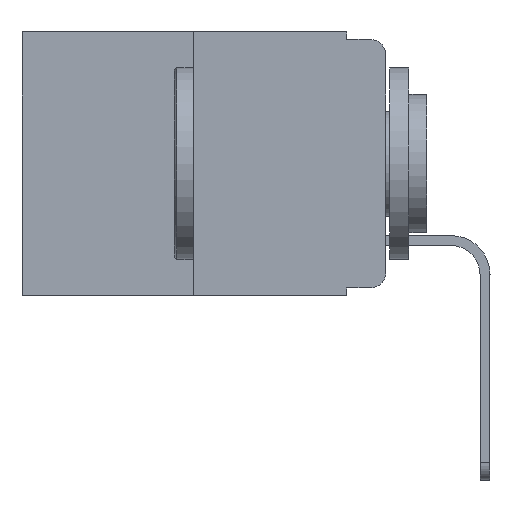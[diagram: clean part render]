
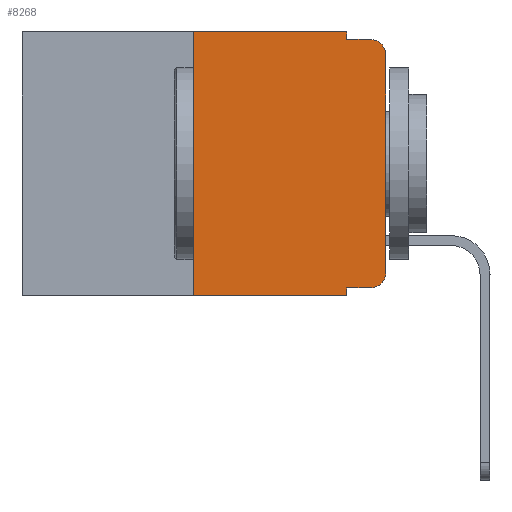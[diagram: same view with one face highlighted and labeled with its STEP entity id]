
A CAD part, left-side view. The second image highlights one B-rep face of the part: STEP entity #8268.
In plain terms, the highlighted planar face has unit normal (-1, 0, 0).
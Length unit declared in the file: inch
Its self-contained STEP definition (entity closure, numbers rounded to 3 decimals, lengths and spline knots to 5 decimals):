
#464 = VERTEX_POINT ( 'NONE', #1537 ) ;
#758 = LINE ( 'NONE', #13825, #1672 ) ;
#880 = CARTESIAN_POINT ( 'NONE',  ( 0., 0.473, 0. ) ) ;
#908 = VERTEX_POINT ( 'NONE', #15043 ) ;
#945 = CARTESIAN_POINT ( 'NONE',  ( 0., 0.02, -0.333 ) ) ;
#1192 = EDGE_CURVE ( 'NONE', #5458, #13924, #758, .T. ) ;
#1350 = DIRECTION ( 'NONE',  ( 0., 0., -1. ) ) ;
#1537 = CARTESIAN_POINT ( 'NONE',  ( 0., 0.25, 0. ) ) ;
#1672 = VECTOR ( 'NONE', #14002, 39.37008 ) ;
#1938 = AXIS2_PLACEMENT_3D ( 'NONE', #14239, #8395, #9851 ) ;
#2137 = VECTOR ( 'NONE', #3473, 39.37008 ) ;
#2298 = EDGE_CURVE ( 'NONE', #14785, #3021, #7307, .T. ) ;
#2560 = EDGE_LOOP ( 'NONE', ( #3801, #17236, #14480, #9229, #12953, #16369, #15485, #13216, #4757, #17441 ) ) ;
#2605 = DIRECTION ( 'NONE',  ( 0., 0., 1. ) ) ;
#2794 = CARTESIAN_POINT ( 'NONE',  ( 0., 0.25, 0. ) ) ;
#3021 = VERTEX_POINT ( 'NONE', #3515 ) ;
#3204 = EDGE_CURVE ( 'NONE', #17879, #13924, #7971, .T. ) ;
#3473 = DIRECTION ( 'NONE',  ( 0., -1., 0. ) ) ;
#3506 = DIRECTION ( 'NONE',  ( 0., 0., 1. ) ) ;
#3515 = CARTESIAN_POINT ( 'NONE',  ( 0., 0.051, -0.01 ) ) ;
#3706 = CARTESIAN_POINT ( 'NONE',  ( 0., 0.051, 0. ) ) ;
#3801 = ORIENTED_EDGE ( 'NONE', *, *, #15115, .T. ) ;
#4421 = CARTESIAN_POINT ( 'NONE',  ( 0., 0.473, 0. ) ) ;
#4757 = ORIENTED_EDGE ( 'NONE', *, *, #10161, .T. ) ;
#4852 = CARTESIAN_POINT ( 'NONE',  ( 0., 0., 0. ) ) ;
#5458 = VERTEX_POINT ( 'NONE', #14608 ) ;
#5532 = LINE ( 'NONE', #880, #13681 ) ;
#5743 = CARTESIAN_POINT ( 'NONE',  ( 0., 0.051, -0.343 ) ) ;
#5960 = EDGE_CURVE ( 'NONE', #908, #10030, #6945, .T. ) ;
#6453 = EDGE_CURVE ( 'NONE', #15244, #16633, #11259, .T. ) ;
#6795 = CARTESIAN_POINT ( 'NONE',  ( 0., 0.473, -0.343 ) ) ;
#6925 = DIRECTION ( 'NONE',  ( 0., -1., 0. ) ) ;
#6945 = CIRCLE ( 'NONE', #8430, 0.02 ) ;
#7133 = DIRECTION ( 'NONE',  ( -1., 0., 0. ) ) ;
#7249 = CARTESIAN_POINT ( 'NONE',  ( 0., 0.051, 0. ) ) ;
#7307 = LINE ( 'NONE', #3706, #8691 ) ;
#7355 = EDGE_CURVE ( 'NONE', #3021, #10030, #13060, .T. ) ;
#7376 = DIRECTION ( 'NONE',  ( 1., 0., 0. ) ) ;
#7581 = FACE_OUTER_BOUND ( 'NONE', #2560, .T. ) ;
#7971 = LINE ( 'NONE', #6795, #17954 ) ;
#8268 = ADVANCED_FACE ( 'NONE', ( #7581 ), #13099, .F. ) ;
#8395 = DIRECTION ( 'NONE',  ( -1., 0., 0. ) ) ;
#8430 = AXIS2_PLACEMENT_3D ( 'NONE', #8550, #7133, #1350 ) ;
#8550 = CARTESIAN_POINT ( 'NONE',  ( 0., 0.02, -0.03 ) ) ;
#8691 = VECTOR ( 'NONE', #10665, 39.37008 ) ;
#9124 = VECTOR ( 'NONE', #15136, 39.37008 ) ;
#9229 = ORIENTED_EDGE ( 'NONE', *, *, #2298, .F. ) ;
#9851 = DIRECTION ( 'NONE',  ( 0., 0., -1. ) ) ;
#10030 = VERTEX_POINT ( 'NONE', #16296 ) ;
#10161 = EDGE_CURVE ( 'NONE', #5458, #15244, #13651, .T. ) ;
#10665 = DIRECTION ( 'NONE',  ( 0., 0., -1. ) ) ;
#11041 = DIRECTION ( 'NONE',  ( 0., -1., 0. ) ) ;
#11259 = CIRCLE ( 'NONE', #1938, 0.02 ) ;
#11471 = VECTOR ( 'NONE', #2605, 39.37008 ) ;
#12383 = CARTESIAN_POINT ( 'NONE',  ( 0., 0.051, -0.333 ) ) ;
#12953 = ORIENTED_EDGE ( 'NONE', *, *, #15248, .F. ) ;
#13060 = LINE ( 'NONE', #13817, #2137 ) ;
#13099 = PLANE ( 'NONE',  #16725 ) ;
#13175 = EDGE_CURVE ( 'NONE', #17879, #464, #17177, .T. ) ;
#13216 = ORIENTED_EDGE ( 'NONE', *, *, #1192, .F. ) ;
#13651 = LINE ( 'NONE', #12383, #9124 ) ;
#13681 = VECTOR ( 'NONE', #11041, 39.37008 ) ;
#13817 = CARTESIAN_POINT ( 'NONE',  ( 0., 0.051, -0.01 ) ) ;
#13825 = CARTESIAN_POINT ( 'NONE',  ( 0., 0.051, 0. ) ) ;
#13924 = VERTEX_POINT ( 'NONE', #5743 ) ;
#14002 = DIRECTION ( 'NONE',  ( 0., 0., -1. ) ) ;
#14239 = CARTESIAN_POINT ( 'NONE',  ( 0., 0.02, -0.313 ) ) ;
#14480 = ORIENTED_EDGE ( 'NONE', *, *, #7355, .F. ) ;
#14572 = DIRECTION ( 'NONE',  ( 0., 0., -1. ) ) ;
#14608 = CARTESIAN_POINT ( 'NONE',  ( 0., 0.051, -0.333 ) ) ;
#14785 = VERTEX_POINT ( 'NONE', #7249 ) ;
#14844 = VECTOR ( 'NONE', #3506, 39.37008 ) ;
#15043 = CARTESIAN_POINT ( 'NONE',  ( 0., 0., -0.03 ) ) ;
#15115 = EDGE_CURVE ( 'NONE', #16633, #908, #17787, .T. ) ;
#15136 = DIRECTION ( 'NONE',  ( 0., -1., 0. ) ) ;
#15244 = VERTEX_POINT ( 'NONE', #945 ) ;
#15248 = EDGE_CURVE ( 'NONE', #464, #14785, #5532, .T. ) ;
#15485 = ORIENTED_EDGE ( 'NONE', *, *, #3204, .T. ) ;
#16296 = CARTESIAN_POINT ( 'NONE',  ( 0., 0.02, -0.01 ) ) ;
#16369 = ORIENTED_EDGE ( 'NONE', *, *, #13175, .F. ) ;
#16633 = VERTEX_POINT ( 'NONE', #18744 ) ;
#16725 = AXIS2_PLACEMENT_3D ( 'NONE', #4421, #7376, #14572 ) ;
#17177 = LINE ( 'NONE', #2794, #11471 ) ;
#17236 = ORIENTED_EDGE ( 'NONE', *, *, #5960, .T. ) ;
#17441 = ORIENTED_EDGE ( 'NONE', *, *, #6453, .T. ) ;
#17787 = LINE ( 'NONE', #4852, #14844 ) ;
#17879 = VERTEX_POINT ( 'NONE', #18489 ) ;
#17954 = VECTOR ( 'NONE', #6925, 39.37008 ) ;
#18489 = CARTESIAN_POINT ( 'NONE',  ( 0., 0.25, -0.343 ) ) ;
#18744 = CARTESIAN_POINT ( 'NONE',  ( 0., 0., -0.313 ) ) ;
